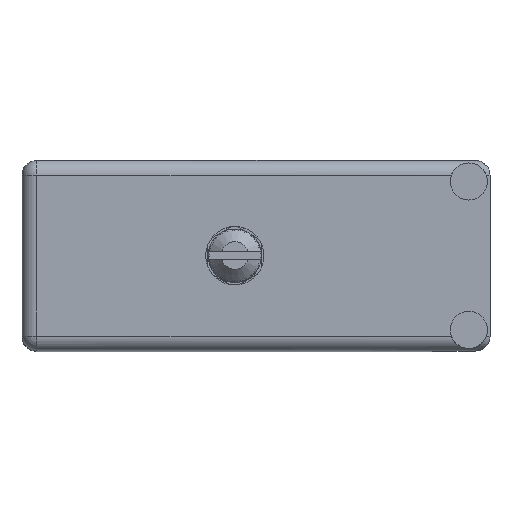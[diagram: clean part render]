
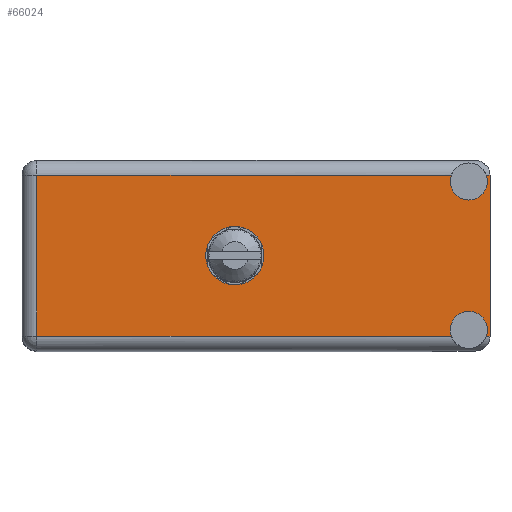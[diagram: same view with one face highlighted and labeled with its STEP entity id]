
A CAD part, top view. The second image highlights one B-rep face of the part: STEP entity #66024.
In plain terms, the highlighted face is planar.
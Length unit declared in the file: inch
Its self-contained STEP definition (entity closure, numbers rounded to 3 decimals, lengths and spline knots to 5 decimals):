
#1450 = EDGE_CURVE ( 'NONE', #14257, #63014, #15353, .T. ) ;
#3255 = DIRECTION ( 'NONE',  ( 0., 1., 0. ) ) ;
#3485 = VERTEX_POINT ( 'NONE', #11381 ) ;
#5794 = VECTOR ( 'NONE', #16994, 39.37008 ) ;
#6582 = CARTESIAN_POINT ( 'NONE',  ( 1.004, 1.566, -0.4495 ) ) ;
#6642 = CARTESIAN_POINT ( 'NONE',  ( 2.108, 1.566, -0.0995 ) ) ;
#7723 = DIRECTION ( 'NONE',  ( 0., 1., 0. ) ) ;
#11381 = CARTESIAN_POINT ( 'NONE',  ( 2.19038, 1.566, -0.829 ) ) ;
#14257 = VERTEX_POINT ( 'NONE', #85776 ) ;
#15353 = LINE ( 'NONE', #34176, #77413 ) ;
#16482 = DIRECTION ( 'NONE',  ( 0., 0., 1. ) ) ;
#16994 = DIRECTION ( 'NONE',  ( -1., 0., 0. ) ) ;
#18764 = CARTESIAN_POINT ( 'NONE',  ( 1.004, 1.566, -0.587 ) ) ;
#20711 = CARTESIAN_POINT ( 'NONE',  ( 2.108, 1.566, -0.712 ) ) ;
#21718 = CARTESIAN_POINT ( 'NONE',  ( 0.07, 1.566, -0.899 ) ) ;
#22039 = DIRECTION ( 'NONE',  ( 0., 0., 1. ) ) ;
#22095 = DIRECTION ( 'NONE',  ( 0., 0., 1. ) ) ;
#22619 = EDGE_CURVE ( 'NONE', #39413, #100012, #110199, .T. ) ;
#23650 = CARTESIAN_POINT ( 'NONE',  ( 2.108, 1.566, -0.7995 ) ) ;
#23836 = CARTESIAN_POINT ( 'NONE',  ( 0., 1.566, -0.899 ) ) ;
#25912 = VECTOR ( 'NONE', #64010, 39.37008 ) ;
#26692 = DIRECTION ( 'NONE',  ( 1., 0., 0. ) ) ;
#26955 = AXIS2_PLACEMENT_3D ( 'NONE', #6642, #84922, #22095 ) ;
#30399 = EDGE_CURVE ( 'NONE', #94098, #39413, #99968, .T. ) ;
#30499 = DIRECTION ( 'NONE',  ( -1., 0., 0. ) ) ;
#31558 = DIRECTION ( 'NONE',  ( 0., 0., 1. ) ) ;
#31829 = DIRECTION ( 'NONE',  ( 0., 0., 1. ) ) ;
#32365 = ORIENTED_EDGE ( 'NONE', *, *, #1450, .F. ) ;
#33192 = ORIENTED_EDGE ( 'NONE', *, *, #36367, .T. ) ;
#34131 = CARTESIAN_POINT ( 'NONE',  ( 0., 1.566, -0.829 ) ) ;
#34176 = CARTESIAN_POINT ( 'NONE',  ( 2.208, 1.566, 0. ) ) ;
#35567 = AXIS2_PLACEMENT_3D ( 'NONE', #57852, #92155, #31558 ) ;
#35992 = CARTESIAN_POINT ( 'NONE',  ( 0.07, 1.566, -0.07 ) ) ;
#36367 = EDGE_CURVE ( 'NONE', #14257, #3485, #48189, .T. ) ;
#37089 = EDGE_CURVE ( 'NONE', #65888, #94098, #60441, .T. ) ;
#39413 = VERTEX_POINT ( 'NONE', #35992 ) ;
#44368 = EDGE_CURVE ( 'NONE', #65888, #51148, #61611, .T. ) ;
#44382 = LINE ( 'NONE', #54082, #55560 ) ;
#45483 = EDGE_CURVE ( 'NONE', #87452, #100012, #76268, .T. ) ;
#45740 = ORIENTED_EDGE ( 'NONE', *, *, #97736, .F. ) ;
#47319 = VERTEX_POINT ( 'NONE', #18764 ) ;
#48013 = ORIENTED_EDGE ( 'NONE', *, *, #75330, .F. ) ;
#48189 = LINE ( 'NONE', #73961, #82495 ) ;
#48836 = CARTESIAN_POINT ( 'NONE',  ( 2.02562, 1.566, -0.07 ) ) ;
#48975 = FACE_BOUND ( 'NONE', #51171, .T. ) ;
#51132 = CARTESIAN_POINT ( 'NONE',  ( 2.108, 1.566, -0.7995 ) ) ;
#51148 = VERTEX_POINT ( 'NONE', #20711 ) ;
#51171 = EDGE_LOOP ( 'NONE', ( #48013, #71787 ) ) ;
#51675 = CARTESIAN_POINT ( 'NONE',  ( 2.19038, 1.566, -0.07 ) ) ;
#53815 = CIRCLE ( 'NONE', #61186, 0.0875 ) ;
#54082 = CARTESIAN_POINT ( 'NONE',  ( 2.208, 1.566, -0.07 ) ) ;
#55560 = VECTOR ( 'NONE', #26692, 39.37008 ) ;
#57116 = CARTESIAN_POINT ( 'NONE',  ( 2.208, 1.566, -0.07 ) ) ;
#57852 = CARTESIAN_POINT ( 'NONE',  ( 2.108, 1.566, -0.0995 ) ) ;
#58351 = EDGE_CURVE ( 'NONE', #51148, #3485, #53815, .T. ) ;
#58997 = VECTOR ( 'NONE', #100536, 39.37008 ) ;
#59192 = ORIENTED_EDGE ( 'NONE', *, *, #22619, .T. ) ;
#59380 = CARTESIAN_POINT ( 'NONE',  ( 2.02562, 1.566, -0.829 ) ) ;
#60441 = LINE ( 'NONE', #34131, #5794 ) ;
#61186 = AXIS2_PLACEMENT_3D ( 'NONE', #51132, #7723, #112789 ) ;
#61611 = CIRCLE ( 'NONE', #79802, 0.0875 ) ;
#61652 = CARTESIAN_POINT ( 'NONE',  ( 2.108, 1.566, -0.187 ) ) ;
#62674 = CIRCLE ( 'NONE', #70038, 0.1375 ) ;
#63014 = VERTEX_POINT ( 'NONE', #88849 ) ;
#64010 = DIRECTION ( 'NONE',  ( 0., 0., 1. ) ) ;
#65888 = VERTEX_POINT ( 'NONE', #59380 ) ;
#66024 = ADVANCED_FACE ( 'NONE', ( #48975, #83851 ), #108384, .T. ) ;
#66104 = CARTESIAN_POINT ( 'NONE',  ( 1.004, 1.566, -0.312 ) ) ;
#66724 = DIRECTION ( 'NONE',  ( 0., 1., 0. ) ) ;
#67710 = AXIS2_PLACEMENT_3D ( 'NONE', #6582, #84859, #22039 ) ;
#69591 = ORIENTED_EDGE ( 'NONE', *, *, #30399, .T. ) ;
#70038 = AXIS2_PLACEMENT_3D ( 'NONE', #98660, #3255, #90685 ) ;
#71787 = ORIENTED_EDGE ( 'NONE', *, *, #110577, .F. ) ;
#73323 = ORIENTED_EDGE ( 'NONE', *, *, #96502, .T. ) ;
#73961 = CARTESIAN_POINT ( 'NONE',  ( 0., 1.566, -0.829 ) ) ;
#75330 = EDGE_CURVE ( 'NONE', #109735, #47319, #84093, .T. ) ;
#76268 = CIRCLE ( 'NONE', #26955, 0.0875 ) ;
#76377 = AXIS2_PLACEMENT_3D ( 'NONE', #23836, #66724, #31829 ) ;
#76524 = ORIENTED_EDGE ( 'NONE', *, *, #45483, .F. ) ;
#77413 = VECTOR ( 'NONE', #16482, 39.37008 ) ;
#77531 = CIRCLE ( 'NONE', #35567, 0.0875 ) ;
#79802 = AXIS2_PLACEMENT_3D ( 'NONE', #23650, #82110, #110428 ) ;
#82110 = DIRECTION ( 'NONE',  ( 0., 1., 0. ) ) ;
#82495 = VECTOR ( 'NONE', #30499, 39.37008 ) ;
#83851 = FACE_OUTER_BOUND ( 'NONE', #101007, .T. ) ;
#84093 = CIRCLE ( 'NONE', #67710, 0.1375 ) ;
#84859 = DIRECTION ( 'NONE',  ( 0., 1., 0. ) ) ;
#84922 = DIRECTION ( 'NONE',  ( 0., 1., 0. ) ) ;
#85776 = CARTESIAN_POINT ( 'NONE',  ( 2.208, 1.566, -0.829 ) ) ;
#85798 = ORIENTED_EDGE ( 'NONE', *, *, #44368, .F. ) ;
#87452 = VERTEX_POINT ( 'NONE', #61652 ) ;
#88475 = VERTEX_POINT ( 'NONE', #51675 ) ;
#88849 = CARTESIAN_POINT ( 'NONE',  ( 2.208, 1.566, -0.07 ) ) ;
#90685 = DIRECTION ( 'NONE',  ( 0., 0., 1. ) ) ;
#92155 = DIRECTION ( 'NONE',  ( 0., 1., 0. ) ) ;
#94098 = VERTEX_POINT ( 'NONE', #104475 ) ;
#96502 = EDGE_CURVE ( 'NONE', #88475, #63014, #44382, .T. ) ;
#97736 = EDGE_CURVE ( 'NONE', #88475, #87452, #77531, .T. ) ;
#98365 = ORIENTED_EDGE ( 'NONE', *, *, #37089, .T. ) ;
#98660 = CARTESIAN_POINT ( 'NONE',  ( 1.004, 1.566, -0.4495 ) ) ;
#99968 = LINE ( 'NONE', #21718, #25912 ) ;
#100012 = VERTEX_POINT ( 'NONE', #48836 ) ;
#100536 = DIRECTION ( 'NONE',  ( 1., 0., 0. ) ) ;
#101007 = EDGE_LOOP ( 'NONE', ( #59192, #76524, #45740, #73323, #32365, #33192, #112155, #85798, #98365, #69591 ) ) ;
#104475 = CARTESIAN_POINT ( 'NONE',  ( 0.07, 1.566, -0.829 ) ) ;
#108384 = PLANE ( 'NONE',  #76377 ) ;
#109735 = VERTEX_POINT ( 'NONE', #66104 ) ;
#110199 = LINE ( 'NONE', #57116, #58997 ) ;
#110428 = DIRECTION ( 'NONE',  ( 0., 0., 1. ) ) ;
#110577 = EDGE_CURVE ( 'NONE', #47319, #109735, #62674, .T. ) ;
#112155 = ORIENTED_EDGE ( 'NONE', *, *, #58351, .F. ) ;
#112789 = DIRECTION ( 'NONE',  ( 0., 0., 1. ) ) ;
